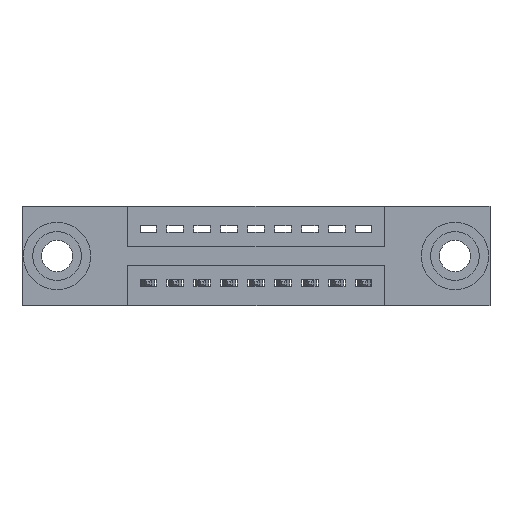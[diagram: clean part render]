
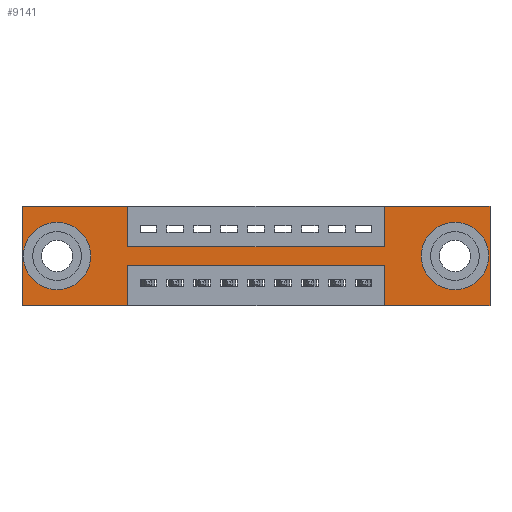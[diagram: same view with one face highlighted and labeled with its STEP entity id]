
A CAD part, front view. The second image highlights one B-rep face of the part: STEP entity #9141.
In plain terms, the highlighted planar face has unit normal (0, -1, 0).
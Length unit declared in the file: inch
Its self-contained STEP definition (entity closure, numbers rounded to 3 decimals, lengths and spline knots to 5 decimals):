
#62 = CARTESIAN_POINT ( 'NONE',  ( 0.13, 0., -0.107 ) ) ;
#135 = PLANE ( 'NONE',  #2839 ) ;
#181 = EDGE_CURVE ( 'NONE', #4426, #9666, #6527, .T. ) ;
#185 = VERTEX_POINT ( 'NONE', #2812 ) ;
#254 = DIRECTION ( 'NONE',  ( 0., 0., 1. ) ) ;
#257 = DIRECTION ( 'NONE',  ( 0., 1., 0. ) ) ;
#264 = FACE_OUTER_BOUND ( 'NONE', #7952, .T. ) ;
#275 = CARTESIAN_POINT ( 'NONE',  ( 0.13, 0., -0.185 ) ) ;
#357 = CIRCLE ( 'NONE', #7005, 0.078 ) ;
#566 = VERTEX_POINT ( 'NONE', #9289 ) ;
#651 = DIRECTION ( 'NONE',  ( 0., 0., 1. ) ) ;
#1211 = CIRCLE ( 'NONE', #9960, 0.078 ) ;
#1216 = DIRECTION ( 'NONE',  ( 0., 0., -1. ) ) ;
#1242 = EDGE_CURVE ( 'NONE', #4256, #2911, #1211, .T. ) ;
#1346 = VECTOR ( 'NONE', #6501, 39.37008 ) ;
#1399 = EDGE_CURVE ( 'NONE', #8357, #2558, #3989, .T. ) ;
#1984 = EDGE_CURVE ( 'NONE', #10950, #8357, #7901, .T. ) ;
#2152 = CARTESIAN_POINT ( 'NONE',  ( 1.605, 0., -0.107 ) ) ;
#2245 = DIRECTION ( 'NONE',  ( 0., 0., -1. ) ) ;
#2272 = LINE ( 'NONE', #11494, #4868 ) ;
#2337 = DIRECTION ( 'NONE',  ( 0., 0., -1. ) ) ;
#2339 = LINE ( 'NONE', #9160, #9336 ) ;
#2407 = VERTEX_POINT ( 'NONE', #4459 ) ;
#2483 = CARTESIAN_POINT ( 'NONE',  ( 0.3925, 0., -0.22 ) ) ;
#2558 = VERTEX_POINT ( 'NONE', #7027 ) ;
#2603 = ORIENTED_EDGE ( 'NONE', *, *, #5498, .T. ) ;
#2733 = ORIENTED_EDGE ( 'NONE', *, *, #1242, .T. ) ;
#2756 = ORIENTED_EDGE ( 'NONE', *, *, #8457, .T. ) ;
#2771 = ORIENTED_EDGE ( 'NONE', *, *, #6443, .T. ) ;
#2798 = ORIENTED_EDGE ( 'NONE', *, *, #3241, .F. ) ;
#2812 = CARTESIAN_POINT ( 'NONE',  ( 0., 0., -0.37 ) ) ;
#2839 = AXIS2_PLACEMENT_3D ( 'NONE', #5956, #6815, #1216 ) ;
#2911 = VERTEX_POINT ( 'NONE', #2152 ) ;
#2956 = CARTESIAN_POINT ( 'NONE',  ( 1.3425, 0., -0.37 ) ) ;
#2966 = LINE ( 'NONE', #3262, #5465 ) ;
#2968 = ORIENTED_EDGE ( 'NONE', *, *, #11544, .F. ) ;
#3069 = VECTOR ( 'NONE', #4530, 39.37008 ) ;
#3082 = ORIENTED_EDGE ( 'NONE', *, *, #1399, .F. ) ;
#3118 = ORIENTED_EDGE ( 'NONE', *, *, #1984, .F. ) ;
#3132 = ORIENTED_EDGE ( 'NONE', *, *, #11561, .F. ) ;
#3241 = EDGE_CURVE ( 'NONE', #11097, #11727, #4982, .T. ) ;
#3262 = CARTESIAN_POINT ( 'NONE',  ( 0.3925, 0., 0. ) ) ;
#3424 = CARTESIAN_POINT ( 'NONE',  ( 0., 0., 0. ) ) ;
#3557 = CARTESIAN_POINT ( 'NONE',  ( 0.3925, 0., -0.37 ) ) ;
#3691 = ORIENTED_EDGE ( 'NONE', *, *, #181, .F. ) ;
#3805 = CARTESIAN_POINT ( 'NONE',  ( 1.3425, 0., -0.15 ) ) ;
#3973 = CARTESIAN_POINT ( 'NONE',  ( 0., 0., -0.37 ) ) ;
#3989 = LINE ( 'NONE', #6496, #1346 ) ;
#4149 = VECTOR ( 'NONE', #651, 39.37008 ) ;
#4174 = VECTOR ( 'NONE', #4950, 39.37008 ) ;
#4212 = CIRCLE ( 'NONE', #11730, 0.078 ) ;
#4222 = VERTEX_POINT ( 'NONE', #62 ) ;
#4228 = DIRECTION ( 'NONE',  ( -1., 0., 0. ) ) ;
#4256 = VERTEX_POINT ( 'NONE', #11751 ) ;
#4398 = DIRECTION ( 'NONE',  ( 0., 0., 1. ) ) ;
#4426 = VERTEX_POINT ( 'NONE', #9015 ) ;
#4459 = CARTESIAN_POINT ( 'NONE',  ( 0.3925, 0., 0. ) ) ;
#4490 = VERTEX_POINT ( 'NONE', #9481 ) ;
#4512 = VECTOR ( 'NONE', #4398, 39.37008 ) ;
#4530 = DIRECTION ( 'NONE',  ( -1., 0., 0. ) ) ;
#4583 = VECTOR ( 'NONE', #2337, 39.37008 ) ;
#4616 = CARTESIAN_POINT ( 'NONE',  ( 1.3425, 0., 0. ) ) ;
#4765 = DIRECTION ( 'NONE',  ( -1., 0., 0. ) ) ;
#4868 = VECTOR ( 'NONE', #5365, 39.37008 ) ;
#4936 = FACE_BOUND ( 'NONE', #5863, .T. ) ;
#4950 = DIRECTION ( 'NONE',  ( 1., 0., 0. ) ) ;
#4982 = LINE ( 'NONE', #9196, #11387 ) ;
#5029 = DIRECTION ( 'NONE',  ( 0., 1., 0. ) ) ;
#5298 = CARTESIAN_POINT ( 'NONE',  ( 0.13, 0., -0.263 ) ) ;
#5365 = DIRECTION ( 'NONE',  ( 1., 0., 0. ) ) ;
#5465 = VECTOR ( 'NONE', #2245, 39.37008 ) ;
#5474 = EDGE_CURVE ( 'NONE', #185, #4490, #9224, .T. ) ;
#5498 = EDGE_CURVE ( 'NONE', #2911, #4256, #4212, .T. ) ;
#5609 = VERTEX_POINT ( 'NONE', #3805 ) ;
#5863 = EDGE_LOOP ( 'NONE', ( #2603, #2733 ) ) ;
#5915 = CARTESIAN_POINT ( 'NONE',  ( 0., 0., 0. ) ) ;
#5956 = CARTESIAN_POINT ( 'NONE',  ( 0., 0., -0.37 ) ) ;
#6021 = CARTESIAN_POINT ( 'NONE',  ( 0.3925, 0., -0.22 ) ) ;
#6443 = EDGE_CURVE ( 'NONE', #10048, #4222, #9885, .T. ) ;
#6496 = CARTESIAN_POINT ( 'NONE',  ( 1.3425, 0., -0.37 ) ) ;
#6501 = DIRECTION ( 'NONE',  ( 0., 0., 1. ) ) ;
#6513 = EDGE_CURVE ( 'NONE', #11727, #185, #2339, .T. ) ;
#6527 = LINE ( 'NONE', #3424, #4174 ) ;
#6625 = LINE ( 'NONE', #7847, #4583 ) ;
#6791 = DIRECTION ( 'NONE',  ( 0., 0., -1. ) ) ;
#6815 = DIRECTION ( 'NONE',  ( 0., -1., 0. ) ) ;
#6841 = CARTESIAN_POINT ( 'NONE',  ( 1.605, 0., -0.185 ) ) ;
#6865 = DIRECTION ( 'NONE',  ( 0., 1., 0. ) ) ;
#7005 = AXIS2_PLACEMENT_3D ( 'NONE', #10298, #5029, #11125 ) ;
#7027 = CARTESIAN_POINT ( 'NONE',  ( 1.3425, 0., -0.22 ) ) ;
#7198 = ORIENTED_EDGE ( 'NONE', *, *, #5474, .F. ) ;
#7320 = ORIENTED_EDGE ( 'NONE', *, *, #9093, .F. ) ;
#7405 = CARTESIAN_POINT ( 'NONE',  ( 1.735, 0., 0. ) ) ;
#7534 = LINE ( 'NONE', #5915, #9901 ) ;
#7558 = ORIENTED_EDGE ( 'NONE', *, *, #9912, .F. ) ;
#7639 = ORIENTED_EDGE ( 'NONE', *, *, #8744, .F. ) ;
#7699 = EDGE_CURVE ( 'NONE', #5609, #4426, #11163, .T. ) ;
#7847 = CARTESIAN_POINT ( 'NONE',  ( 1.735, 0., 0. ) ) ;
#7901 = LINE ( 'NONE', #3973, #3069 ) ;
#7952 = EDGE_LOOP ( 'NONE', ( #2798, #2968, #3082, #3118, #3132, #3691, #8499, #7639, #7558, #7320, #7198, #8052 ) ) ;
#8052 = ORIENTED_EDGE ( 'NONE', *, *, #6513, .F. ) ;
#8357 = VERTEX_POINT ( 'NONE', #2956 ) ;
#8457 = EDGE_CURVE ( 'NONE', #4222, #10048, #357, .T. ) ;
#8499 = ORIENTED_EDGE ( 'NONE', *, *, #7699, .F. ) ;
#8635 = CARTESIAN_POINT ( 'NONE',  ( 1.735, 0., -0.37 ) ) ;
#8744 = EDGE_CURVE ( 'NONE', #566, #5609, #2272, .T. ) ;
#8769 = DIRECTION ( 'NONE',  ( 0., 0., -1. ) ) ;
#8819 = DIRECTION ( 'NONE',  ( 0., 1., 0. ) ) ;
#8840 = CARTESIAN_POINT ( 'NONE',  ( 1.605, 0., -0.185 ) ) ;
#8992 = DIRECTION ( 'NONE',  ( 0., 0., -1. ) ) ;
#9015 = CARTESIAN_POINT ( 'NONE',  ( 1.3425, 0., 0. ) ) ;
#9093 = EDGE_CURVE ( 'NONE', #4490, #2407, #7534, .T. ) ;
#9141 = ADVANCED_FACE ( 'NONE', ( #4936, #9631, #264 ), #135, .T. ) ;
#9160 = CARTESIAN_POINT ( 'NONE',  ( 0., 0., -0.37 ) ) ;
#9180 = AXIS2_PLACEMENT_3D ( 'NONE', #275, #257, #254 ) ;
#9196 = CARTESIAN_POINT ( 'NONE',  ( 0.3925, 0., -0.37 ) ) ;
#9224 = LINE ( 'NONE', #10958, #4512 ) ;
#9289 = CARTESIAN_POINT ( 'NONE',  ( 0.3925, 0., -0.15 ) ) ;
#9336 = VECTOR ( 'NONE', #4765, 39.37008 ) ;
#9481 = CARTESIAN_POINT ( 'NONE',  ( 0., 0., 0. ) ) ;
#9566 = LINE ( 'NONE', #6021, #11537 ) ;
#9631 = FACE_BOUND ( 'NONE', #10800, .T. ) ;
#9666 = VERTEX_POINT ( 'NONE', #7405 ) ;
#9885 = CIRCLE ( 'NONE', #9180, 0.078 ) ;
#9901 = VECTOR ( 'NONE', #11149, 39.37008 ) ;
#9912 = EDGE_CURVE ( 'NONE', #2407, #566, #2966, .T. ) ;
#9960 = AXIS2_PLACEMENT_3D ( 'NONE', #8840, #8819, #8769 ) ;
#10048 = VERTEX_POINT ( 'NONE', #5298 ) ;
#10298 = CARTESIAN_POINT ( 'NONE',  ( 0.13, 0., -0.185 ) ) ;
#10800 = EDGE_LOOP ( 'NONE', ( #2756, #2771 ) ) ;
#10950 = VERTEX_POINT ( 'NONE', #8635 ) ;
#10958 = CARTESIAN_POINT ( 'NONE',  ( 0., 0., 0. ) ) ;
#11097 = VERTEX_POINT ( 'NONE', #2483 ) ;
#11125 = DIRECTION ( 'NONE',  ( 0., 0., 1. ) ) ;
#11149 = DIRECTION ( 'NONE',  ( 1., 0., 0. ) ) ;
#11163 = LINE ( 'NONE', #4616, #4149 ) ;
#11387 = VECTOR ( 'NONE', #8992, 39.37008 ) ;
#11494 = CARTESIAN_POINT ( 'NONE',  ( 0.3925, 0., -0.15 ) ) ;
#11537 = VECTOR ( 'NONE', #4228, 39.37008 ) ;
#11544 = EDGE_CURVE ( 'NONE', #2558, #11097, #9566, .T. ) ;
#11561 = EDGE_CURVE ( 'NONE', #9666, #10950, #6625, .T. ) ;
#11727 = VERTEX_POINT ( 'NONE', #3557 ) ;
#11730 = AXIS2_PLACEMENT_3D ( 'NONE', #6841, #6865, #6791 ) ;
#11751 = CARTESIAN_POINT ( 'NONE',  ( 1.605, 0., -0.263 ) ) ;
